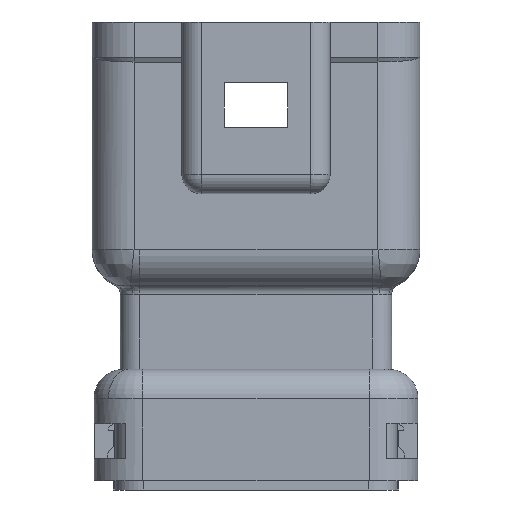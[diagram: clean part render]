
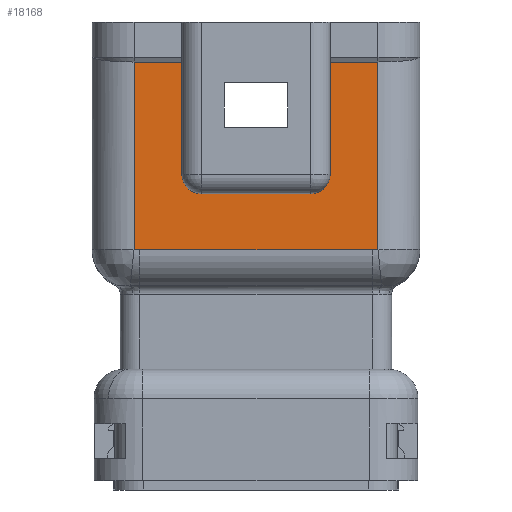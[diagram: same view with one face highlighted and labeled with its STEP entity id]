
A CAD part, front view. The second image highlights one B-rep face of the part: STEP entity #18168.
In plain terms, the highlighted planar face has unit normal (0, -1, 0).
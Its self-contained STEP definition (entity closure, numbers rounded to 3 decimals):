
#11 = LINE ( 'NONE', #32977, #22932 ) ;
#123 = DIRECTION ( 'NONE',  ( 0., 0., 1. ) ) ;
#321 = EDGE_CURVE ( 'NONE', #20113, #29344, #976, .T. ) ;
#676 = CARTESIAN_POINT ( 'NONE',  ( 14.65, 2.2, -12.341 ) ) ;
#976 = LINE ( 'NONE', #27925, #33272 ) ;
#1304 = ORIENTED_EDGE ( 'NONE', *, *, #27221, .F. ) ;
#2764 = CARTESIAN_POINT ( 'NONE',  ( 4.6, 2.2, -21.93 ) ) ;
#3157 = DIRECTION ( 'NONE',  ( 0., 0., 1. ) ) ;
#3220 = VERTEX_POINT ( 'NONE', #27435 ) ;
#3382 = CARTESIAN_POINT ( 'NONE',  ( 2.211, 2.2, -12.335 ) ) ;
#3401 = CARTESIAN_POINT ( 'NONE',  ( 14.436, 2.2, -12.324 ) ) ;
#3592 = CARTESIAN_POINT ( 'NONE',  ( 14.638, 2.2, -12.339 ) ) ;
#4031 = VERTEX_POINT ( 'NONE', #18724 ) ;
#4282 = VECTOR ( 'NONE', #3157, 1000. ) ;
#4606 =( BOUNDED_CURVE ( )  B_SPLINE_CURVE ( 3, ( #18408, #24283, #3382, #24478, #27216, #30315, #21341 ),
 .UNSPECIFIED., .F., .F. ) 
 B_SPLINE_CURVE_WITH_KNOTS ( ( 4, 1, 1, 1, 4 ),
 ( 0., 0.141, 0.419, 0.707, 1. ),
 .UNSPECIFIED. ) 
 CURVE ( )  GEOMETRIC_REPRESENTATION_ITEM ( )  RATIONAL_B_SPLINE_CURVE ( ( 1.098, 1.098, 1.098, 1.098, 1.098, 1.098, 1.098 ) ) 
 REPRESENTATION_ITEM ( '' )  );
#4792 = ORIENTED_EDGE ( 'NONE', *, *, #321, .F. ) ;
#5464 = LINE ( 'NONE', #13672, #31909 ) ;
#7442 = PLANE ( 'NONE',  #21576 ) ;
#7733 = VERTEX_POINT ( 'NONE', #9480 ) ;
#8036 = EDGE_CURVE ( 'NONE', #18675, #21902, #4606, .T. ) ;
#8411 = EDGE_CURVE ( 'NONE', #28059, #29344, #23481, .T. ) ;
#8749 = CARTESIAN_POINT ( 'NONE',  ( 14.65, 2.2, -12.341 ) ) ;
#9186 = EDGE_CURVE ( 'NONE', #13147, #7733, #20570, .T. ) ;
#9380 = CARTESIAN_POINT ( 'NONE',  ( 5.6, 2.2, -15.18 ) ) ;
#9384 = DIRECTION ( 'NONE',  ( 0., 1., 0. ) ) ;
#9456 = CARTESIAN_POINT ( 'NONE',  ( 14.524, 2.2, -12.329 ) ) ;
#9474 = EDGE_CURVE ( 'NONE', #17334, #38209, #14120, .T. ) ;
#9480 = CARTESIAN_POINT ( 'NONE',  ( 4.6, 2.2, -21.93 ) ) ;
#9554 = CARTESIAN_POINT ( 'NONE',  ( 14.65, 2.2, -21.93 ) ) ;
#9911 = EDGE_CURVE ( 'NONE', #7733, #28059, #17203, .T. ) ;
#9930 = LINE ( 'NONE', #36474, #22237 ) ;
#10477 = ORIENTED_EDGE ( 'NONE', *, *, #31229, .F. ) ;
#11215 = DIRECTION ( 'NONE',  ( 0., 0., 1. ) ) ;
#11378 = ORIENTED_EDGE ( 'NONE', *, *, #36478, .F. ) ;
#11995 = CARTESIAN_POINT ( 'NONE',  ( 14.35, 2.2, -12.323 ) ) ;
#12586 = ORIENTED_EDGE ( 'NONE', *, *, #8411, .T. ) ;
#12879 = AXIS2_PLACEMENT_3D ( 'NONE', #24432, #9384, #36313 ) ;
#13147 = VERTEX_POINT ( 'NONE', #15047 ) ;
#13434 = CARTESIAN_POINT ( 'NONE',  ( 12.2, 2.2, -16.18 ) ) ;
#13435 = ORIENTED_EDGE ( 'NONE', *, *, #24587, .T. ) ;
#13672 = CARTESIAN_POINT ( 'NONE',  ( 2.45, 2.2, -12.323 ) ) ;
#13677 = CARTESIAN_POINT ( 'NONE',  ( 2.15, 2.2, -21.93 ) ) ;
#14120 = LINE ( 'NONE', #26066, #31071 ) ;
#14905 = DIRECTION ( 'NONE',  ( 1., 0., 0. ) ) ;
#15047 = CARTESIAN_POINT ( 'NONE',  ( 2.15, 2.2, -21.93 ) ) ;
#15430 = AXIS2_PLACEMENT_3D ( 'NONE', #34746, #24519, #28207 ) ;
#17203 = LINE ( 'NONE', #2764, #4282 ) ;
#17319 = VECTOR ( 'NONE', #14905, 1000. ) ;
#17334 = VERTEX_POINT ( 'NONE', #9554 ) ;
#17418 = ORIENTED_EDGE ( 'NONE', *, *, #22507, .F. ) ;
#18168 = ADVANCED_FACE ( 'NONE', ( #34559 ), #7442, .T. ) ;
#18408 = CARTESIAN_POINT ( 'NONE',  ( 2.15, 2.2, -12.341 ) ) ;
#18675 = VERTEX_POINT ( 'NONE', #20074 ) ;
#18724 = CARTESIAN_POINT ( 'NONE',  ( 14.35, 2.2, -12.323 ) ) ;
#18741 = DIRECTION ( 'NONE',  ( 1., 0., 0. ) ) ;
#20074 = CARTESIAN_POINT ( 'NONE',  ( 2.15, 2.2, -12.341 ) ) ;
#20113 = VERTEX_POINT ( 'NONE', #30613 ) ;
#20570 = LINE ( 'NONE', #37614, #17319 ) ;
#21341 = CARTESIAN_POINT ( 'NONE',  ( 2.45, 2.2, -12.323 ) ) ;
#21576 = AXIS2_PLACEMENT_3D ( 'NONE', #13677, #25617, #37297 ) ;
#21902 = VERTEX_POINT ( 'NONE', #32825 ) ;
#22237 = VECTOR ( 'NONE', #33935, 1000. ) ;
#22507 = EDGE_CURVE ( 'NONE', #13147, #18675, #9930, .T. ) ;
#22584 = ORIENTED_EDGE ( 'NONE', *, *, #8036, .F. ) ;
#22932 = VECTOR ( 'NONE', #18741, 1000. ) ;
#23481 = CIRCLE ( 'NONE', #12879, 1. ) ;
#23649 = EDGE_CURVE ( 'NONE', #3220, #17334, #11, .T. ) ;
#23998 = ORIENTED_EDGE ( 'NONE', *, *, #9911, .T. ) ;
#24283 = CARTESIAN_POINT ( 'NONE',  ( 2.166, 2.2, -12.339 ) ) ;
#24432 = CARTESIAN_POINT ( 'NONE',  ( 5.6, 2.2, -16.18 ) ) ;
#24435 = DIRECTION ( 'NONE',  ( -1., 0., 0. ) ) ;
#24478 = CARTESIAN_POINT ( 'NONE',  ( 2.284, 2.2, -12.328 ) ) ;
#24519 = DIRECTION ( 'NONE',  ( 0., 1., 0. ) ) ;
#24575 = ORIENTED_EDGE ( 'NONE', *, *, #9186, .T. ) ;
#24587 = EDGE_CURVE ( 'NONE', #20113, #38017, #27877, .T. ) ;
#25617 = DIRECTION ( 'NONE',  ( 0., -1., 0. ) ) ;
#26066 = CARTESIAN_POINT ( 'NONE',  ( 14.65, 2.2, -21.93 ) ) ;
#26892 = CARTESIAN_POINT ( 'NONE',  ( 12.2, 2.2, -21.93 ) ) ;
#27216 = CARTESIAN_POINT ( 'NONE',  ( 2.368, 2.2, -12.324 ) ) ;
#27221 = EDGE_CURVE ( 'NONE', #4031, #38209, #32304, .T. ) ;
#27435 = CARTESIAN_POINT ( 'NONE',  ( 12.2, 2.2, -21.93 ) ) ;
#27442 = CARTESIAN_POINT ( 'NONE',  ( 14.595, 2.2, -12.335 ) ) ;
#27524 = VECTOR ( 'NONE', #123, 1000. ) ;
#27877 = CIRCLE ( 'NONE', #15430, 1. ) ;
#27925 = CARTESIAN_POINT ( 'NONE',  ( 11.2, 2.2, -15.18 ) ) ;
#28059 = VERTEX_POINT ( 'NONE', #36083 ) ;
#28207 = DIRECTION ( 'NONE',  ( 0., 0., 1. ) ) ;
#29344 = VERTEX_POINT ( 'NONE', #9380 ) ;
#30315 = CARTESIAN_POINT ( 'NONE',  ( 2.422, 2.2, -12.323 ) ) ;
#30339 = CARTESIAN_POINT ( 'NONE',  ( 14.379, 2.2, -12.323 ) ) ;
#30613 = CARTESIAN_POINT ( 'NONE',  ( 11.2, 2.2, -15.18 ) ) ;
#31071 = VECTOR ( 'NONE', #11215, 1000. ) ;
#31229 = EDGE_CURVE ( 'NONE', #3220, #38017, #35246, .T. ) ;
#31909 = VECTOR ( 'NONE', #34554, 1000. ) ;
#32304 =( BOUNDED_CURVE ( )  B_SPLINE_CURVE ( 3, ( #11995, #30339, #3401, #9456, #27442, #3592, #676 ),
 .UNSPECIFIED., .F., .F. ) 
 B_SPLINE_CURVE_WITH_KNOTS ( ( 4, 1, 1, 1, 4 ),
 ( 0., 0.307, 0.606, 0.895, 1. ),
 .UNSPECIFIED. ) 
 CURVE ( )  GEOMETRIC_REPRESENTATION_ITEM ( )  RATIONAL_B_SPLINE_CURVE ( ( 1.098, 1.098, 1.098, 1.098, 1.098, 1.098, 1.098 ) ) 
 REPRESENTATION_ITEM ( '' )  );
#32318 = ORIENTED_EDGE ( 'NONE', *, *, #9474, .T. ) ;
#32825 = CARTESIAN_POINT ( 'NONE',  ( 2.45, 2.2, -12.323 ) ) ;
#32977 = CARTESIAN_POINT ( 'NONE',  ( 12.2, 2.2, -21.93 ) ) ;
#33272 = VECTOR ( 'NONE', #24435, 1000. ) ;
#33935 = DIRECTION ( 'NONE',  ( 0., 0., 1. ) ) ;
#34455 = ORIENTED_EDGE ( 'NONE', *, *, #23649, .T. ) ;
#34554 = DIRECTION ( 'NONE',  ( 1., 0., 0. ) ) ;
#34559 = FACE_OUTER_BOUND ( 'NONE', #38066, .T. ) ;
#34746 = CARTESIAN_POINT ( 'NONE',  ( 11.2, 2.2, -16.18 ) ) ;
#35246 = LINE ( 'NONE', #26892, #27524 ) ;
#36083 = CARTESIAN_POINT ( 'NONE',  ( 4.6, 2.2, -16.18 ) ) ;
#36313 = DIRECTION ( 'NONE',  ( -1., 0., 0. ) ) ;
#36474 = CARTESIAN_POINT ( 'NONE',  ( 2.15, 2.2, -21.93 ) ) ;
#36478 = EDGE_CURVE ( 'NONE', #21902, #4031, #5464, .T. ) ;
#37297 = DIRECTION ( 'NONE',  ( 1., 0., 0. ) ) ;
#37614 = CARTESIAN_POINT ( 'NONE',  ( 2.15, 2.2, -21.93 ) ) ;
#38017 = VERTEX_POINT ( 'NONE', #13434 ) ;
#38066 = EDGE_LOOP ( 'NONE', ( #13435, #10477, #34455, #32318, #1304, #11378, #22584, #17418, #24575, #23998, #12586, #4792 ) ) ;
#38209 = VERTEX_POINT ( 'NONE', #8749 ) ;
